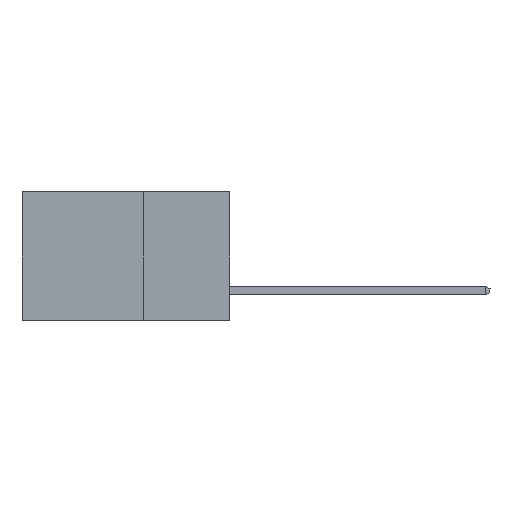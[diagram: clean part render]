
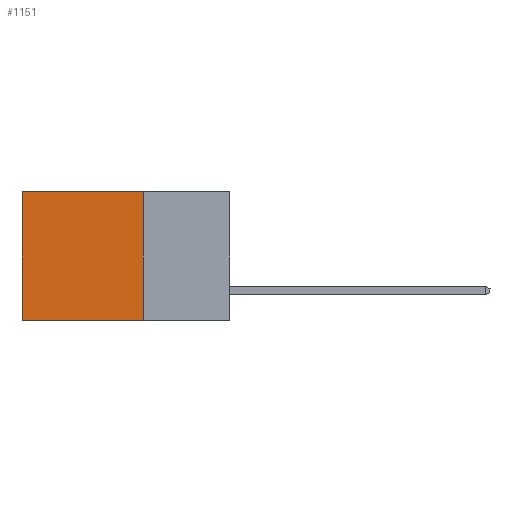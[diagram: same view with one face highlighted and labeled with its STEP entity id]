
A CAD part, left-side view. The second image highlights one B-rep face of the part: STEP entity #1151.
In plain terms, the highlighted planar face has unit normal (-1, 0, 0).
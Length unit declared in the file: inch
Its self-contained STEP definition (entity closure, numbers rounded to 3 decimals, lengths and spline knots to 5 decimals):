
#706 = VERTEX_POINT ( 'NONE', #11809 ) ;
#1151 = ADVANCED_FACE ( 'NONE', ( #13795 ), #9334, .F. ) ;
#1491 = DIRECTION ( 'NONE',  ( 1., 0., 0. ) ) ;
#1807 = ORIENTED_EDGE ( 'NONE', *, *, #6800, .T. ) ;
#2382 = DIRECTION ( 'NONE',  ( 0., 0., -1. ) ) ;
#2559 = EDGE_LOOP ( 'NONE', ( #12808, #9890, #9022, #1807 ) ) ;
#2571 = LINE ( 'NONE', #6922, #11244 ) ;
#3238 = CARTESIAN_POINT ( 'NONE',  ( 0.2615, 0.25, -0.37 ) ) ;
#3555 = CARTESIAN_POINT ( 'NONE',  ( 0.2615, 0.6, -0.37 ) ) ;
#3772 = VECTOR ( 'NONE', #11211, 39.37008 ) ;
#3815 = VECTOR ( 'NONE', #13272, 39.37008 ) ;
#3819 = DIRECTION ( 'NONE',  ( 0., 0., -1. ) ) ;
#4458 = EDGE_CURVE ( 'NONE', #706, #13662, #6752, .T. ) ;
#4513 = CARTESIAN_POINT ( 'NONE',  ( 0.2615, 0.25, -0.37 ) ) ;
#5648 = VERTEX_POINT ( 'NONE', #6225 ) ;
#5741 = LINE ( 'NONE', #6614, #3815 ) ;
#6225 = CARTESIAN_POINT ( 'NONE',  ( 0.2615, 0.6, -0.37 ) ) ;
#6473 = CARTESIAN_POINT ( 'NONE',  ( 0.2615, 0.6, 0. ) ) ;
#6553 = EDGE_CURVE ( 'NONE', #13662, #5648, #2571, .T. ) ;
#6614 = CARTESIAN_POINT ( 'NONE',  ( 0.2615, 0.25, 0. ) ) ;
#6752 = LINE ( 'NONE', #4513, #3772 ) ;
#6800 = EDGE_CURVE ( 'NONE', #706, #9862, #5741, .T. ) ;
#6922 = CARTESIAN_POINT ( 'NONE',  ( 0.2615, 0.25, -0.37 ) ) ;
#8021 = DIRECTION ( 'NONE',  ( 0., 1., 0. ) ) ;
#9022 = ORIENTED_EDGE ( 'NONE', *, *, #4458, .F. ) ;
#9266 = CARTESIAN_POINT ( 'NONE',  ( 0.2615, 0.25, -0.37 ) ) ;
#9334 = PLANE ( 'NONE',  #14151 ) ;
#9862 = VERTEX_POINT ( 'NONE', #6473 ) ;
#9890 = ORIENTED_EDGE ( 'NONE', *, *, #6553, .F. ) ;
#10381 = EDGE_CURVE ( 'NONE', #9862, #5648, #12509, .T. ) ;
#11211 = DIRECTION ( 'NONE',  ( 0., 0., -1. ) ) ;
#11244 = VECTOR ( 'NONE', #8021, 39.37008 ) ;
#11809 = CARTESIAN_POINT ( 'NONE',  ( 0.2615, 0.25, 0. ) ) ;
#12423 = VECTOR ( 'NONE', #2382, 39.37008 ) ;
#12509 = LINE ( 'NONE', #3555, #12423 ) ;
#12808 = ORIENTED_EDGE ( 'NONE', *, *, #10381, .T. ) ;
#13272 = DIRECTION ( 'NONE',  ( 0., 1., 0. ) ) ;
#13662 = VERTEX_POINT ( 'NONE', #3238 ) ;
#13795 = FACE_OUTER_BOUND ( 'NONE', #2559, .T. ) ;
#14151 = AXIS2_PLACEMENT_3D ( 'NONE', #9266, #1491, #3819 ) ;
